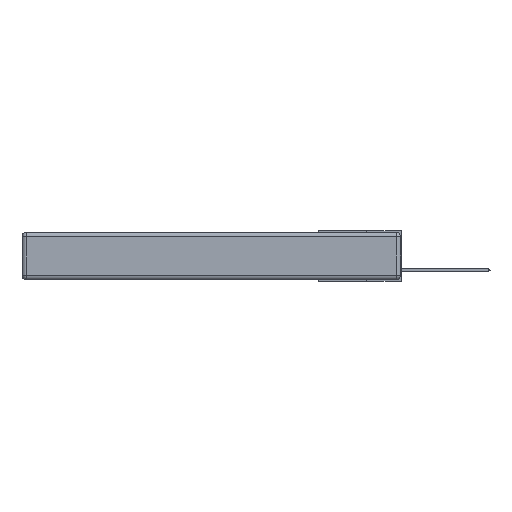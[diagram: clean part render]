
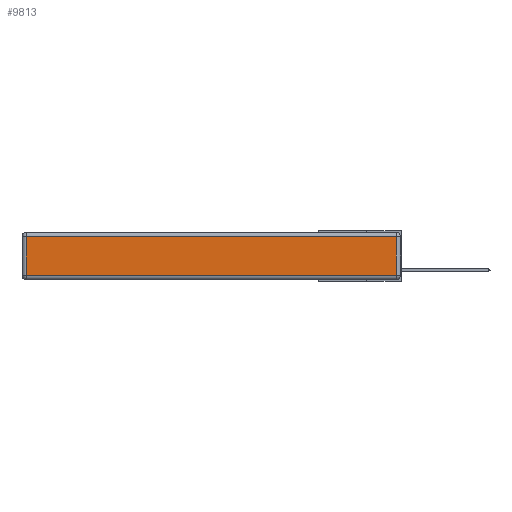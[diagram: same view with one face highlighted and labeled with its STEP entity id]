
A CAD part, left-side view. The second image highlights one B-rep face of the part: STEP entity #9813.
In plain terms, the highlighted planar face has unit normal (-1, 0, 0).
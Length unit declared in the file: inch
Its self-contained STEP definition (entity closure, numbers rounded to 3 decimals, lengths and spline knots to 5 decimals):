
#2441 = ORIENTED_EDGE ( 'NONE', *, *, #16767, .T. ) ;
#3679 = VERTEX_POINT ( 'NONE', #29615 ) ;
#4000 = LINE ( 'NONE', #26127, #23788 ) ;
#5390 = VERTEX_POINT ( 'NONE', #28291 ) ;
#5431 = VERTEX_POINT ( 'NONE', #14973 ) ;
#6215 = FACE_OUTER_BOUND ( 'NONE', #16390, .T. ) ;
#6809 = EDGE_CURVE ( 'NONE', #3679, #26829, #4000, .T. ) ;
#6986 = ORIENTED_EDGE ( 'NONE', *, *, #8179, .T. ) ;
#7190 = VECTOR ( 'NONE', #10467, 39.37008 ) ;
#8179 = EDGE_CURVE ( 'NONE', #5431, #3679, #11576, .T. ) ;
#9813 = ADVANCED_FACE ( 'NONE', ( #6215 ), #14468, .T. ) ;
#10467 = DIRECTION ( 'NONE',  ( 0., 0., -1. ) ) ;
#11189 = VECTOR ( 'NONE', #21113, 39.37008 ) ;
#11576 = LINE ( 'NONE', #18412, #11189 ) ;
#14162 = CARTESIAN_POINT ( 'NONE',  ( 0., 2.72, -0.03 ) ) ;
#14468 = PLANE ( 'NONE',  #28019 ) ;
#14973 = CARTESIAN_POINT ( 'NONE',  ( 0., 0.03, -0.313 ) ) ;
#16390 = EDGE_LOOP ( 'NONE', ( #2441, #6986, #26613, #21413 ) ) ;
#16767 = EDGE_CURVE ( 'NONE', #5390, #5431, #29153, .T. ) ;
#17906 = CARTESIAN_POINT ( 'NONE',  ( 0., 2.72, -0.343 ) ) ;
#18412 = CARTESIAN_POINT ( 'NONE',  ( 0., 0.03, -0.343 ) ) ;
#20259 = EDGE_CURVE ( 'NONE', #26829, #5390, #27747, .T. ) ;
#20712 = VECTOR ( 'NONE', #23390, 39.37008 ) ;
#21113 = DIRECTION ( 'NONE',  ( 0., 0., 1. ) ) ;
#21413 = ORIENTED_EDGE ( 'NONE', *, *, #20259, .T. ) ;
#21947 = DIRECTION ( 'NONE',  ( -1., 0., 0. ) ) ;
#23390 = DIRECTION ( 'NONE',  ( 0., -1., 0. ) ) ;
#23788 = VECTOR ( 'NONE', #28517, 39.37008 ) ;
#26127 = CARTESIAN_POINT ( 'NONE',  ( 0., 2.75, -0.03 ) ) ;
#26613 = ORIENTED_EDGE ( 'NONE', *, *, #6809, .T. ) ;
#26829 = VERTEX_POINT ( 'NONE', #14162 ) ;
#26888 = CARTESIAN_POINT ( 'NONE',  ( 0., 0., -0.343 ) ) ;
#27114 = DIRECTION ( 'NONE',  ( 0., 0., 1. ) ) ;
#27747 = LINE ( 'NONE', #17906, #7190 ) ;
#28019 = AXIS2_PLACEMENT_3D ( 'NONE', #26888, #21947, #27114 ) ;
#28291 = CARTESIAN_POINT ( 'NONE',  ( 0., 2.72, -0.313 ) ) ;
#28517 = DIRECTION ( 'NONE',  ( 0., 1., 0. ) ) ;
#29153 = LINE ( 'NONE', #31024, #20712 ) ;
#29615 = CARTESIAN_POINT ( 'NONE',  ( 0., 0.03, -0.03 ) ) ;
#31024 = CARTESIAN_POINT ( 'NONE',  ( 0., 0., -0.313 ) ) ;
